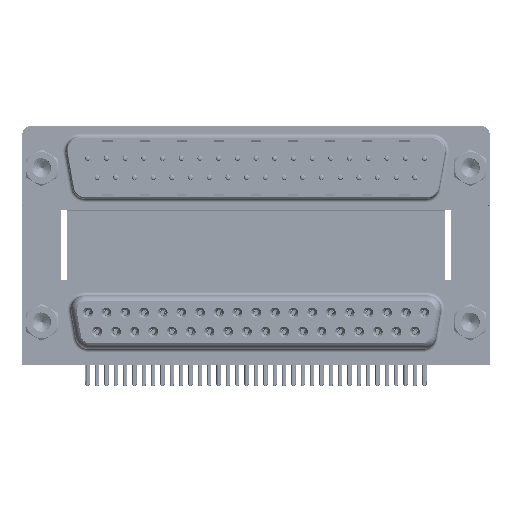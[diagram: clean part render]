
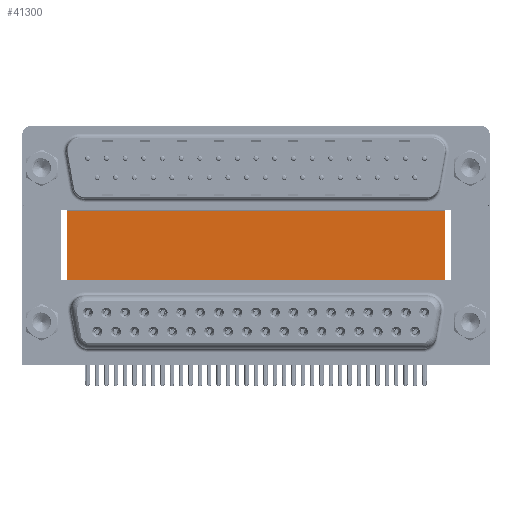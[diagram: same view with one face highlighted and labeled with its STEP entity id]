
A CAD part, top view. The second image highlights one B-rep face of the part: STEP entity #41300.
In plain terms, the highlighted planar face has unit normal (0, 0, 1).
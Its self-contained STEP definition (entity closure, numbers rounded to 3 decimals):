
#4039 = DIRECTION ( 'NONE',  ( 1., 0., 0. ) ) ;
#5050 = EDGE_CURVE ( 'NONE', #49091, #57519, #50899, .T. ) ;
#8642 = AXIS2_PLACEMENT_3D ( 'NONE', #27783, #38420, #66290 ) ;
#9939 = CARTESIAN_POINT ( 'NONE',  ( 3.79, 16.585, -12. ) ) ;
#10142 = EDGE_CURVE ( 'NONE', #52096, #49091, #53922, .T. ) ;
#20560 = ORIENTED_EDGE ( 'NONE', *, *, #10142, .F. ) ;
#20595 = CARTESIAN_POINT ( 'NONE',  ( 3.79, 16.585, -12. ) ) ;
#27783 = CARTESIAN_POINT ( 'NONE',  ( 3.79, 16.585, -12. ) ) ;
#27842 = VECTOR ( 'NONE', #4039, 1000. ) ;
#29259 = DIRECTION ( 'NONE',  ( 0., -1., 0. ) ) ;
#29856 = DIRECTION ( 'NONE',  ( 1., 0., 0. ) ) ;
#32047 = CARTESIAN_POINT ( 'NONE',  ( 3.79, -3.735, -12. ) ) ;
#32567 = PLANE ( 'NONE',  #8642 ) ;
#32983 = CARTESIAN_POINT ( 'NONE',  ( 3.79, 16.585, -12. ) ) ;
#33614 = VECTOR ( 'NONE', #29856, 1000. ) ;
#36200 = EDGE_LOOP ( 'NONE', ( #36774, #40170, #20560, #39542 ) ) ;
#36774 = ORIENTED_EDGE ( 'NONE', *, *, #63092, .T. ) ;
#38420 = DIRECTION ( 'NONE',  ( 0., 0., -1. ) ) ;
#38544 = VECTOR ( 'NONE', #52519, 1000. ) ;
#39542 = ORIENTED_EDGE ( 'NONE', *, *, #51923, .T. ) ;
#40170 = ORIENTED_EDGE ( 'NONE', *, *, #5050, .F. ) ;
#40868 = CARTESIAN_POINT ( 'NONE',  ( 3.79, -3.735, -12. ) ) ;
#41300 = ADVANCED_FACE ( 'NONE', ( #60822 ), #32567, .F. ) ;
#42963 = VERTEX_POINT ( 'NONE', #32047 ) ;
#49091 = VERTEX_POINT ( 'NONE', #61281 ) ;
#50899 = LINE ( 'NONE', #62629, #61378 ) ;
#51923 = EDGE_CURVE ( 'NONE', #52096, #42963, #69728, .T. ) ;
#52096 = VERTEX_POINT ( 'NONE', #9939 ) ;
#52519 = DIRECTION ( 'NONE',  ( 0., -1., 0. ) ) ;
#53922 = LINE ( 'NONE', #32983, #27842 ) ;
#55594 = CARTESIAN_POINT ( 'NONE',  ( 59.71, -3.735, -12. ) ) ;
#57519 = VERTEX_POINT ( 'NONE', #55594 ) ;
#60822 = FACE_OUTER_BOUND ( 'NONE', #36200, .T. ) ;
#61281 = CARTESIAN_POINT ( 'NONE',  ( 59.71, 16.585, -12. ) ) ;
#61378 = VECTOR ( 'NONE', #29259, 1000. ) ;
#62629 = CARTESIAN_POINT ( 'NONE',  ( 59.71, 16.585, -12. ) ) ;
#63092 = EDGE_CURVE ( 'NONE', #42963, #57519, #63597, .T. ) ;
#63597 = LINE ( 'NONE', #40868, #33614 ) ;
#66290 = DIRECTION ( 'NONE',  ( -1., 0., 0. ) ) ;
#69728 = LINE ( 'NONE', #20595, #38544 ) ;
